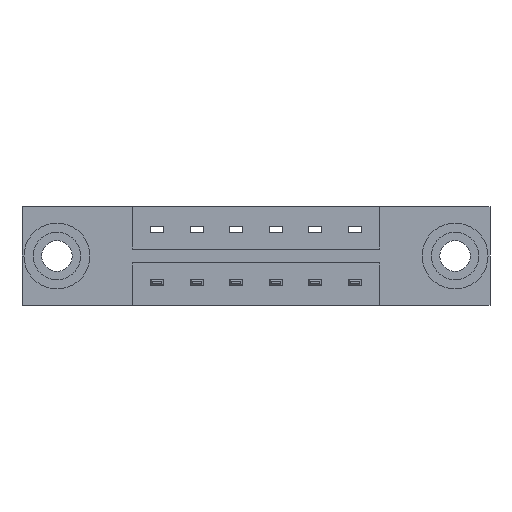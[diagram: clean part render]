
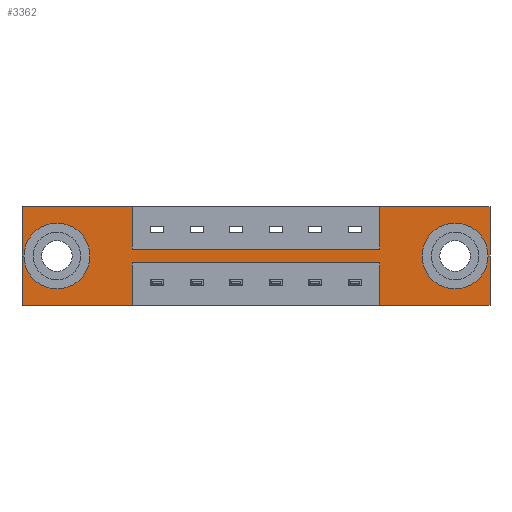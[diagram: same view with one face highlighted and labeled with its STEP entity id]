
A CAD part, front view. The second image highlights one B-rep face of the part: STEP entity #3362.
In plain terms, the highlighted planar face has unit normal (0, -1, 0).
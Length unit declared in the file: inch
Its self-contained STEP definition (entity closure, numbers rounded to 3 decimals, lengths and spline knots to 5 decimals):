
#1 = CARTESIAN_POINT ( 'NONE',  ( 0.4175, 0., -0.161 ) ) ;
#29 = CIRCLE ( 'NONE', #7643, 0.078 ) ;
#74 = CARTESIAN_POINT ( 'NONE',  ( 0.1325, 0., -0.1875 ) ) ;
#111 = ORIENTED_EDGE ( 'NONE', *, *, #5547, .F. ) ;
#184 = CARTESIAN_POINT ( 'NONE',  ( 1.775, 0., 0. ) ) ;
#313 = VECTOR ( 'NONE', #6061, 39.37008 ) ;
#368 = EDGE_CURVE ( 'NONE', #6868, #8598, #29, .T. ) ;
#574 = DIRECTION ( 'NONE',  ( 1., 0., 0. ) ) ;
#578 = CIRCLE ( 'NONE', #4631, 0.078 ) ;
#638 = DIRECTION ( 'NONE',  ( 0., 0., 1. ) ) ;
#687 = CARTESIAN_POINT ( 'NONE',  ( 0.4175, 0., -0.214 ) ) ;
#708 = EDGE_CURVE ( 'NONE', #8310, #8709, #578, .T. ) ;
#728 = ORIENTED_EDGE ( 'NONE', *, *, #6726, .T. ) ;
#738 = VECTOR ( 'NONE', #5067, 39.37008 ) ;
#753 = CARTESIAN_POINT ( 'NONE',  ( 0.4175, 0., -0.214 ) ) ;
#823 = LINE ( 'NONE', #687, #3448 ) ;
#875 = CARTESIAN_POINT ( 'NONE',  ( 0., 0., -0.375 ) ) ;
#898 = LINE ( 'NONE', #184, #7881 ) ;
#1049 = ORIENTED_EDGE ( 'NONE', *, *, #3179, .F. ) ;
#1051 = CARTESIAN_POINT ( 'NONE',  ( 1.775, 0., 0. ) ) ;
#1062 = VECTOR ( 'NONE', #5304, 39.37008 ) ;
#1123 = VECTOR ( 'NONE', #6027, 39.37008 ) ;
#1240 = EDGE_CURVE ( 'NONE', #3835, #1394, #3013, .T. ) ;
#1371 = CARTESIAN_POINT ( 'NONE',  ( 0.1325, 0., -0.2655 ) ) ;
#1394 = VERTEX_POINT ( 'NONE', #4250 ) ;
#1431 = DIRECTION ( 'NONE',  ( 0., 0., -1. ) ) ;
#1723 = VERTEX_POINT ( 'NONE', #3805 ) ;
#2104 = VERTEX_POINT ( 'NONE', #875 ) ;
#2111 = CARTESIAN_POINT ( 'NONE',  ( 0.4175, 0., 0. ) ) ;
#2128 = VECTOR ( 'NONE', #574, 39.37008 ) ;
#2152 = DIRECTION ( 'NONE',  ( 0., 0., -1. ) ) ;
#2176 = CARTESIAN_POINT ( 'NONE',  ( 0.4175, 0., -0.375 ) ) ;
#2189 = DIRECTION ( 'NONE',  ( 0., 1., 0. ) ) ;
#2197 = LINE ( 'NONE', #4459, #738 ) ;
#2207 = CARTESIAN_POINT ( 'NONE',  ( 0., 0., 0. ) ) ;
#2249 = AXIS2_PLACEMENT_3D ( 'NONE', #7523, #8211, #6236 ) ;
#2262 = CARTESIAN_POINT ( 'NONE',  ( 0.4175, 0., -0.161 ) ) ;
#2293 = LINE ( 'NONE', #7046, #7502 ) ;
#2418 = LINE ( 'NONE', #1, #2933 ) ;
#2500 = EDGE_CURVE ( 'NONE', #8186, #8096, #823, .T. ) ;
#2667 = VECTOR ( 'NONE', #1431, 39.37008 ) ;
#2775 = CARTESIAN_POINT ( 'NONE',  ( 1.3575, 0., -0.214 ) ) ;
#2861 = EDGE_LOOP ( 'NONE', ( #5872, #111, #5148, #5060, #5787, #6337, #4999, #3028, #2901, #7214, #1049, #5874 ) ) ;
#2881 = LINE ( 'NONE', #753, #2667 ) ;
#2888 = EDGE_CURVE ( 'NONE', #1394, #8013, #3754, .T. ) ;
#2901 = ORIENTED_EDGE ( 'NONE', *, *, #6780, .F. ) ;
#2933 = VECTOR ( 'NONE', #4137, 39.37008 ) ;
#3013 = LINE ( 'NONE', #2262, #6745 ) ;
#3028 = ORIENTED_EDGE ( 'NONE', *, *, #8425, .F. ) ;
#3084 = LINE ( 'NONE', #7363, #2128 ) ;
#3101 = FACE_OUTER_BOUND ( 'NONE', #2861, .T. ) ;
#3179 = EDGE_CURVE ( 'NONE', #8096, #6478, #2881, .T. ) ;
#3258 = EDGE_CURVE ( 'NONE', #5881, #5540, #898, .T. ) ;
#3275 = DIRECTION ( 'NONE',  ( 0., 1., 0. ) ) ;
#3359 = VERTEX_POINT ( 'NONE', #2207 ) ;
#3362 = ADVANCED_FACE ( 'NONE', ( #8632, #6729, #3101 ), #4835, .T. ) ;
#3388 = CARTESIAN_POINT ( 'NONE',  ( 1.6425, 0., -0.1875 ) ) ;
#3448 = VECTOR ( 'NONE', #4041, 39.37008 ) ;
#3515 = DIRECTION ( 'NONE',  ( 1., 0., 0. ) ) ;
#3563 = ORIENTED_EDGE ( 'NONE', *, *, #368, .T. ) ;
#3644 = VECTOR ( 'NONE', #638, 39.37008 ) ;
#3692 = CIRCLE ( 'NONE', #4644, 0.078 ) ;
#3754 = LINE ( 'NONE', #7981, #3644 ) ;
#3805 = CARTESIAN_POINT ( 'NONE',  ( 1.3575, 0., -0.375 ) ) ;
#3835 = VERTEX_POINT ( 'NONE', #8550 ) ;
#3888 = EDGE_CURVE ( 'NONE', #8013, #5881, #3084, .T. ) ;
#3999 = EDGE_LOOP ( 'NONE', ( #3563, #8104 ) ) ;
#4041 = DIRECTION ( 'NONE',  ( -1., 0., 0. ) ) ;
#4137 = DIRECTION ( 'NONE',  ( 0., 0., -1. ) ) ;
#4219 = AXIS2_PLACEMENT_3D ( 'NONE', #74, #6945, #6978 ) ;
#4250 = CARTESIAN_POINT ( 'NONE',  ( 1.3575, 0., -0.161 ) ) ;
#4349 = DIRECTION ( 'NONE',  ( 0., 1., 0. ) ) ;
#4381 = CARTESIAN_POINT ( 'NONE',  ( 0.1325, 0., -0.1875 ) ) ;
#4459 = CARTESIAN_POINT ( 'NONE',  ( 0., 0., 0. ) ) ;
#4631 = AXIS2_PLACEMENT_3D ( 'NONE', #3388, #3275, #8077 ) ;
#4644 = AXIS2_PLACEMENT_3D ( 'NONE', #5602, #2189, #6950 ) ;
#4678 = CARTESIAN_POINT ( 'NONE',  ( 0., 0., 0. ) ) ;
#4835 = PLANE ( 'NONE',  #2249 ) ;
#4898 = EDGE_CURVE ( 'NONE', #1723, #8186, #6688, .T. ) ;
#4903 = CARTESIAN_POINT ( 'NONE',  ( 0.4175, 0., -0.214 ) ) ;
#4999 = ORIENTED_EDGE ( 'NONE', *, *, #6719, .F. ) ;
#5060 = ORIENTED_EDGE ( 'NONE', *, *, #3888, .F. ) ;
#5067 = DIRECTION ( 'NONE',  ( 0., 0., 1. ) ) ;
#5148 = ORIENTED_EDGE ( 'NONE', *, *, #3258, .F. ) ;
#5304 = DIRECTION ( 'NONE',  ( -1., 0., 0. ) ) ;
#5398 = CARTESIAN_POINT ( 'NONE',  ( 1.6425, 0., -0.1095 ) ) ;
#5427 = CARTESIAN_POINT ( 'NONE',  ( 0., 0., -0.375 ) ) ;
#5540 = VERTEX_POINT ( 'NONE', #8800 ) ;
#5547 = EDGE_CURVE ( 'NONE', #5540, #1723, #6680, .T. ) ;
#5602 = CARTESIAN_POINT ( 'NONE',  ( 1.6425, 0., -0.1875 ) ) ;
#5787 = ORIENTED_EDGE ( 'NONE', *, *, #2888, .F. ) ;
#5872 = ORIENTED_EDGE ( 'NONE', *, *, #4898, .F. ) ;
#5874 = ORIENTED_EDGE ( 'NONE', *, *, #2500, .F. ) ;
#5881 = VERTEX_POINT ( 'NONE', #1051 ) ;
#6027 = DIRECTION ( 'NONE',  ( 1., 0., 0. ) ) ;
#6061 = DIRECTION ( 'NONE',  ( 0., 0., 1. ) ) ;
#6236 = DIRECTION ( 'NONE',  ( 0., 0., -1. ) ) ;
#6337 = ORIENTED_EDGE ( 'NONE', *, *, #1240, .F. ) ;
#6420 = EDGE_LOOP ( 'NONE', ( #728, #6814 ) ) ;
#6443 = LINE ( 'NONE', #4678, #1123 ) ;
#6476 = CIRCLE ( 'NONE', #4219, 0.078 ) ;
#6478 = VERTEX_POINT ( 'NONE', #2176 ) ;
#6564 = EDGE_CURVE ( 'NONE', #8598, #6868, #6476, .T. ) ;
#6680 = LINE ( 'NONE', #5427, #1062 ) ;
#6688 = LINE ( 'NONE', #7506, #313 ) ;
#6715 = CARTESIAN_POINT ( 'NONE',  ( 0.1325, 0., -0.1095 ) ) ;
#6719 = EDGE_CURVE ( 'NONE', #6986, #3835, #2418, .T. ) ;
#6726 = EDGE_CURVE ( 'NONE', #8709, #8310, #3692, .T. ) ;
#6729 = FACE_BOUND ( 'NONE', #3999, .T. ) ;
#6745 = VECTOR ( 'NONE', #3515, 39.37008 ) ;
#6780 = EDGE_CURVE ( 'NONE', #2104, #3359, #2197, .T. ) ;
#6814 = ORIENTED_EDGE ( 'NONE', *, *, #708, .T. ) ;
#6868 = VERTEX_POINT ( 'NONE', #6715 ) ;
#6945 = DIRECTION ( 'NONE',  ( 0., 1., 0. ) ) ;
#6950 = DIRECTION ( 'NONE',  ( 0., 0., -1. ) ) ;
#6978 = DIRECTION ( 'NONE',  ( 0., 0., 1. ) ) ;
#6986 = VERTEX_POINT ( 'NONE', #2111 ) ;
#7019 = DIRECTION ( 'NONE',  ( -1., 0., 0. ) ) ;
#7046 = CARTESIAN_POINT ( 'NONE',  ( 0., 0., -0.375 ) ) ;
#7121 = DIRECTION ( 'NONE',  ( 0., 0., 1. ) ) ;
#7190 = CARTESIAN_POINT ( 'NONE',  ( 1.6425, 0., -0.2655 ) ) ;
#7214 = ORIENTED_EDGE ( 'NONE', *, *, #7612, .F. ) ;
#7363 = CARTESIAN_POINT ( 'NONE',  ( 0., 0., 0. ) ) ;
#7502 = VECTOR ( 'NONE', #7019, 39.37008 ) ;
#7506 = CARTESIAN_POINT ( 'NONE',  ( 1.3575, 0., -0.214 ) ) ;
#7523 = CARTESIAN_POINT ( 'NONE',  ( 0., 0., -0.375 ) ) ;
#7612 = EDGE_CURVE ( 'NONE', #6478, #2104, #2293, .T. ) ;
#7643 = AXIS2_PLACEMENT_3D ( 'NONE', #4381, #4349, #7121 ) ;
#7881 = VECTOR ( 'NONE', #2152, 39.37008 ) ;
#7981 = CARTESIAN_POINT ( 'NONE',  ( 1.3575, 0., -0.161 ) ) ;
#8013 = VERTEX_POINT ( 'NONE', #8733 ) ;
#8077 = DIRECTION ( 'NONE',  ( 0., 0., -1. ) ) ;
#8096 = VERTEX_POINT ( 'NONE', #4903 ) ;
#8104 = ORIENTED_EDGE ( 'NONE', *, *, #6564, .T. ) ;
#8186 = VERTEX_POINT ( 'NONE', #2775 ) ;
#8211 = DIRECTION ( 'NONE',  ( 0., -1., 0. ) ) ;
#8310 = VERTEX_POINT ( 'NONE', #7190 ) ;
#8425 = EDGE_CURVE ( 'NONE', #3359, #6986, #6443, .T. ) ;
#8550 = CARTESIAN_POINT ( 'NONE',  ( 0.4175, 0., -0.161 ) ) ;
#8598 = VERTEX_POINT ( 'NONE', #1371 ) ;
#8632 = FACE_BOUND ( 'NONE', #6420, .T. ) ;
#8709 = VERTEX_POINT ( 'NONE', #5398 ) ;
#8733 = CARTESIAN_POINT ( 'NONE',  ( 1.3575, 0., 0. ) ) ;
#8800 = CARTESIAN_POINT ( 'NONE',  ( 1.775, 0., -0.375 ) ) ;
